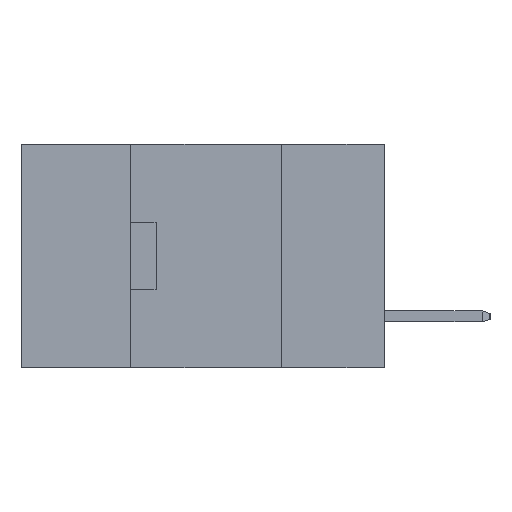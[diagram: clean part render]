
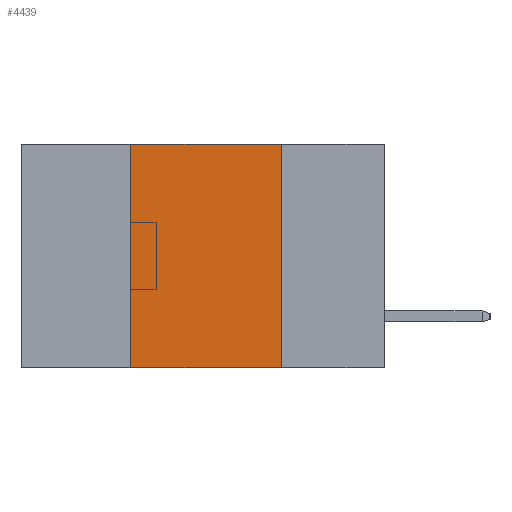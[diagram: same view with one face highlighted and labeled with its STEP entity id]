
A CAD part, left-side view. The second image highlights one B-rep face of the part: STEP entity #4439.
In plain terms, the highlighted planar face has unit normal (-1, 0, 0).
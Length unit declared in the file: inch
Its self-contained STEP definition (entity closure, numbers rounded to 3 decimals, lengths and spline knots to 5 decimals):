
#163 = VECTOR ( 'NONE', #21545, 39.37008 ) ;
#1271 = CARTESIAN_POINT ( 'NONE',  ( 0., 0.6, 0. ) ) ;
#1367 = ORIENTED_EDGE ( 'NONE', *, *, #4446, .T. ) ;
#3804 = LINE ( 'NONE', #15721, #14301 ) ;
#4063 = VERTEX_POINT ( 'NONE', #26958 ) ;
#4439 = ADVANCED_FACE ( 'NONE', ( #20621 ), #7596, .F. ) ;
#4446 = EDGE_CURVE ( 'NONE', #24016, #25482, #9482, .T. ) ;
#5638 = DIRECTION ( 'NONE',  ( 0., 0., 1. ) ) ;
#6527 = CARTESIAN_POINT ( 'NONE',  ( 0., 0.42, 0. ) ) ;
#7476 = CARTESIAN_POINT ( 'NONE',  ( 0., 0.42, -0.37 ) ) ;
#7596 = PLANE ( 'NONE',  #9654 ) ;
#8634 = ORIENTED_EDGE ( 'NONE', *, *, #13751, .F. ) ;
#9005 = CARTESIAN_POINT ( 'NONE',  ( 0., 0.6, 0. ) ) ;
#9482 = LINE ( 'NONE', #18030, #19961 ) ;
#9654 = AXIS2_PLACEMENT_3D ( 'NONE', #1271, #22240, #9709 ) ;
#9709 = DIRECTION ( 'NONE',  ( 0., 0., -1. ) ) ;
#11066 = CARTESIAN_POINT ( 'NONE',  ( 0., 0.17, -0.37 ) ) ;
#11242 = EDGE_LOOP ( 'NONE', ( #22017, #24335, #8634, #1367 ) ) ;
#12334 = VECTOR ( 'NONE', #5638, 39.37008 ) ;
#13621 = EDGE_CURVE ( 'NONE', #4063, #25482, #3804, .T. ) ;
#13751 = EDGE_CURVE ( 'NONE', #24016, #19676, #17893, .T. ) ;
#14301 = VECTOR ( 'NONE', #17839, 39.37008 ) ;
#15721 = CARTESIAN_POINT ( 'NONE',  ( 0., 0.17, -0.37 ) ) ;
#17839 = DIRECTION ( 'NONE',  ( 0., 0., -1. ) ) ;
#17893 = LINE ( 'NONE', #24403, #12334 ) ;
#18030 = CARTESIAN_POINT ( 'NONE',  ( 0., 0.6, -0.37 ) ) ;
#19676 = VERTEX_POINT ( 'NONE', #6527 ) ;
#19803 = EDGE_CURVE ( 'NONE', #19676, #4063, #21783, .T. ) ;
#19961 = VECTOR ( 'NONE', #20236, 39.37008 ) ;
#20236 = DIRECTION ( 'NONE',  ( 0., -1., 0. ) ) ;
#20621 = FACE_OUTER_BOUND ( 'NONE', #11242, .T. ) ;
#21545 = DIRECTION ( 'NONE',  ( 0., -1., 0. ) ) ;
#21783 = LINE ( 'NONE', #9005, #163 ) ;
#22017 = ORIENTED_EDGE ( 'NONE', *, *, #13621, .F. ) ;
#22240 = DIRECTION ( 'NONE',  ( 1., 0., 0. ) ) ;
#24016 = VERTEX_POINT ( 'NONE', #7476 ) ;
#24335 = ORIENTED_EDGE ( 'NONE', *, *, #19803, .F. ) ;
#24403 = CARTESIAN_POINT ( 'NONE',  ( 0., 0.42, -0.37 ) ) ;
#25482 = VERTEX_POINT ( 'NONE', #11066 ) ;
#26958 = CARTESIAN_POINT ( 'NONE',  ( 0., 0.17, 0. ) ) ;
